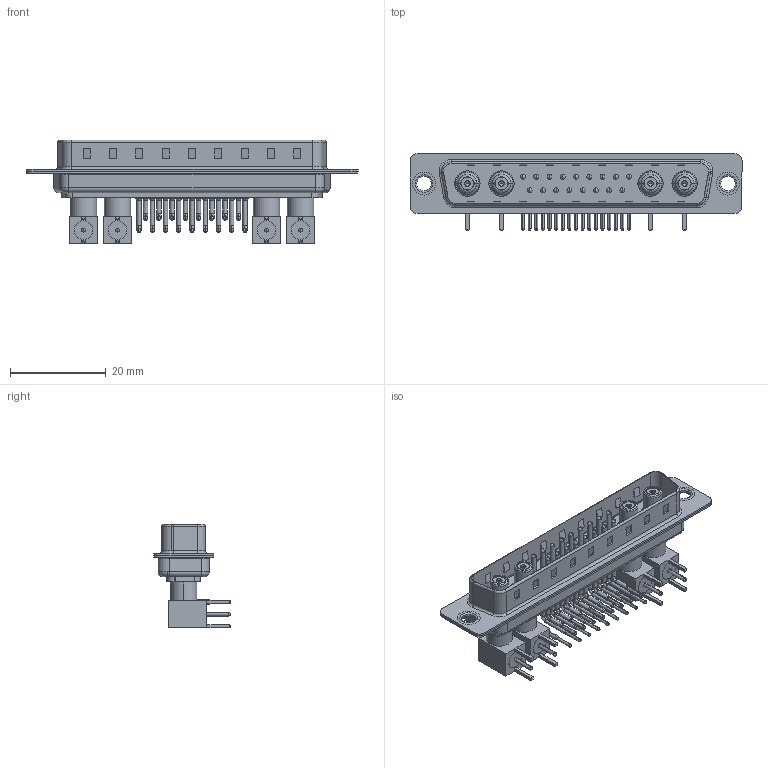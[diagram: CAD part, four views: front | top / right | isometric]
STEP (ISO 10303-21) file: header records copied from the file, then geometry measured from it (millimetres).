
FILE_DESCRIPTION (( 'STEP AP203' ), '1' );
FILE_NAME ('629-21W4240-7N1.STEP', '2022-05-17T01:43:46', ( '' ), ( '' ), 'SwSTEP 2.0', 'SolidWorks 2020', '' );
FILE_SCHEMA (( 'CONFIG_CONTROL_DESIGN' ));
Length unit declared in the file: millimetre
Products named in the file (18): Co-Ax Jack Assy_RA; 629Combo Thru Hole Rivet; 629Combo Shell Front_37 Contacts; 629Combo Shell Rear_37 Contacts; Locking Collar; 629Combo Contact Row 1; RA Back Shell; 629-21W4240-7N1; 629Combo Housing_21W4; 629Combo Contact Row 2; Insulator Socket 2; Insulator Socket; Insulator RA Pin; Socket_RA; Co-Ax Jack_RA PC Tail
Assembly tree (54 placements, depth 3):
  629-21W4240-7N1
    629Combo Housing_21W4
    629Combo Shell Rear_37 Contacts
    629Combo Shell Front_37 Contacts
    629Combo Thru Hole Rivet  x2
    Co-Ax Jack Assy_RA
      Co-Ax Jack_RA PC Tail
      Insulator Socket
      Insulator Socket 2
      Locking Collar
      Socket_RA
      RA Back Shell
      Insulator RA Pin
    Co-Ax Jack Assy_RA
      Co-Ax Jack_RA PC Tail
      Insulator Socket
      Insulator Socket 2
      Locking Collar
      Socket_RA
      RA Back Shell
      Insulator RA Pin
    Co-Ax Jack Assy_RA
      Co-Ax Jack_RA PC Tail
      Insulator Socket
      Insulator Socket 2
      Locking Collar
      Socket_RA
      RA Back Shell
      Insulator RA Pin
    Co-Ax Jack Assy_RA
      Co-Ax Jack_RA PC Tail
      Insulator Socket
      Insulator Socket 2
      Locking Collar
      Socket_RA
      RA Back Shell
      Insulator RA Pin
    629Combo Contact Row 1  x9
    629Combo Contact Row 2  x8
Bounding box: 69.4 x 16 x 21.71 mm (x, y, z)
Volume: 4971.1 mm3; surface area: 13341.1 mm2
Topology: 50 solids, 50 shells, 2864 faces, 7643 edges, 4914 vertices
Faces by surface type: plane 1519, cylinder 1005, cone 144, bspline 106, torus 82, sphere 8
Entity records: 29807 total; most frequent: CARTESIAN_POINT 4968, DIRECTION 4837, ORIENTED_EDGE 4376, EDGE_CURVE 2188, AXIS2_PLACEMENT_3D 1761, VERTEX_POINT 1407, LINE 1315, VECTOR 1315
